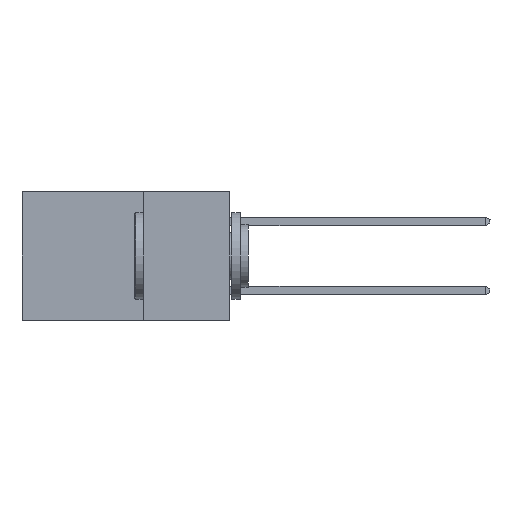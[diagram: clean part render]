
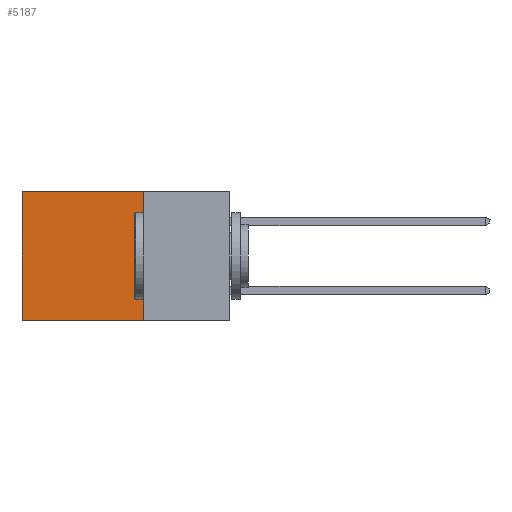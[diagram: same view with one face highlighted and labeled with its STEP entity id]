
A CAD part, left-side view. The second image highlights one B-rep face of the part: STEP entity #5187.
In plain terms, the highlighted planar face has unit normal (-1, 0, 0).
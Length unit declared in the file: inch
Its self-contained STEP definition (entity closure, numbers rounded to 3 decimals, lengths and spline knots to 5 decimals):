
#26 = VERTEX_POINT ( 'NONE', #18295 ) ;
#45 = EDGE_LOOP ( 'NONE', ( #12632, #11811, #5825, #16034 ) ) ;
#328 = VERTEX_POINT ( 'NONE', #21221 ) ;
#925 = AXIS2_PLACEMENT_3D ( 'NONE', #1427, #8676, #8078 ) ;
#1031 = CARTESIAN_POINT ( 'NONE',  ( 0.298, 0.25, 0. ) ) ;
#1395 = CARTESIAN_POINT ( 'NONE',  ( 0.298, 0.25, 0. ) ) ;
#1427 = CARTESIAN_POINT ( 'NONE',  ( 0.298, 0.25, 0. ) ) ;
#2297 = VECTOR ( 'NONE', #10896, 39.37008 ) ;
#3357 = LINE ( 'NONE', #1395, #20753 ) ;
#3924 = DIRECTION ( 'NONE',  ( 0., 1., 0. ) ) ;
#5187 = ADVANCED_FACE ( 'NONE', ( #7079 ), #19436, .F. ) ;
#5825 = ORIENTED_EDGE ( 'NONE', *, *, #9869, .F. ) ;
#5835 = CARTESIAN_POINT ( 'NONE',  ( 0.298, 0.6, 0. ) ) ;
#6050 = CARTESIAN_POINT ( 'NONE',  ( 0.298, 0.25, -0.37 ) ) ;
#6720 = CARTESIAN_POINT ( 'NONE',  ( 0.298, 0.25, 0. ) ) ;
#6930 = VECTOR ( 'NONE', #14804, 39.37008 ) ;
#7079 = FACE_OUTER_BOUND ( 'NONE', #45, .T. ) ;
#8078 = DIRECTION ( 'NONE',  ( 0., 0., -1. ) ) ;
#8676 = DIRECTION ( 'NONE',  ( 1., 0., 0. ) ) ;
#9869 = EDGE_CURVE ( 'NONE', #15280, #12937, #3357, .T. ) ;
#10896 = DIRECTION ( 'NONE',  ( 0., 0., -1. ) ) ;
#11389 = LINE ( 'NONE', #1031, #6930 ) ;
#11738 = VECTOR ( 'NONE', #3924, 39.37008 ) ;
#11811 = ORIENTED_EDGE ( 'NONE', *, *, #13496, .F. ) ;
#12282 = LINE ( 'NONE', #17430, #11738 ) ;
#12632 = ORIENTED_EDGE ( 'NONE', *, *, #21992, .T. ) ;
#12937 = VERTEX_POINT ( 'NONE', #6050 ) ;
#13496 = EDGE_CURVE ( 'NONE', #12937, #26, #12282, .T. ) ;
#14804 = DIRECTION ( 'NONE',  ( 0., 1., 0. ) ) ;
#15121 = EDGE_CURVE ( 'NONE', #15280, #328, #11389, .T. ) ;
#15133 = DIRECTION ( 'NONE',  ( 0., 0., -1. ) ) ;
#15280 = VERTEX_POINT ( 'NONE', #6720 ) ;
#15425 = LINE ( 'NONE', #5835, #2297 ) ;
#16034 = ORIENTED_EDGE ( 'NONE', *, *, #15121, .T. ) ;
#17430 = CARTESIAN_POINT ( 'NONE',  ( 0.298, 0.25, -0.37 ) ) ;
#18295 = CARTESIAN_POINT ( 'NONE',  ( 0.298, 0.6, -0.37 ) ) ;
#19436 = PLANE ( 'NONE',  #925 ) ;
#20753 = VECTOR ( 'NONE', #15133, 39.37008 ) ;
#21221 = CARTESIAN_POINT ( 'NONE',  ( 0.298, 0.6, 0. ) ) ;
#21992 = EDGE_CURVE ( 'NONE', #328, #26, #15425, .T. ) ;
